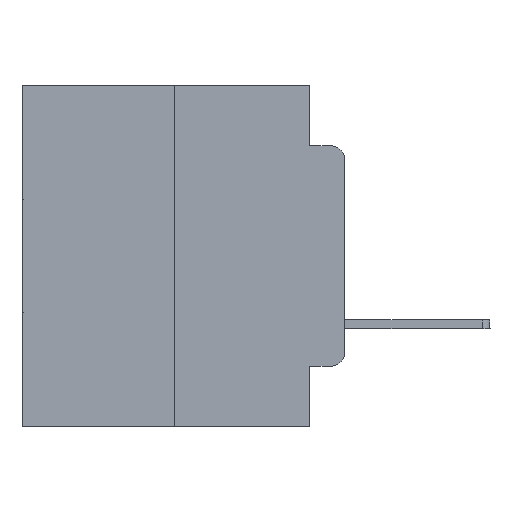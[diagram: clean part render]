
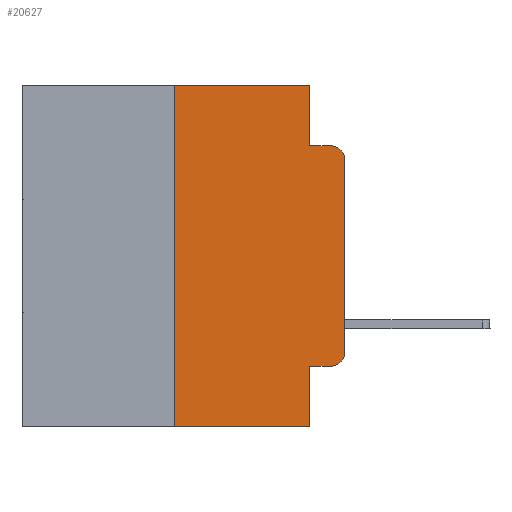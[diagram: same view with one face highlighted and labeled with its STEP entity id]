
A CAD part, left-side view. The second image highlights one B-rep face of the part: STEP entity #20627.
In plain terms, the highlighted planar face has unit normal (-1, 0, 0).
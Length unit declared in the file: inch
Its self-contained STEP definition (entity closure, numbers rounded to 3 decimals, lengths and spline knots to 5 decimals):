
#305 = ORIENTED_EDGE ( 'NONE', *, *, #5010, .T. ) ;
#1034 = ORIENTED_EDGE ( 'NONE', *, *, #11892, .F. ) ;
#1563 = CARTESIAN_POINT ( 'NONE',  ( 0., 0.02, -0.0885 ) ) ;
#1621 = ORIENTED_EDGE ( 'NONE', *, *, #8146, .T. ) ;
#1834 = ORIENTED_EDGE ( 'NONE', *, *, #20499, .T. ) ;
#1839 = VECTOR ( 'NONE', #17886, 39.37008 ) ;
#2283 = DIRECTION ( 'NONE',  ( 0., -1., 0. ) ) ;
#2463 = CARTESIAN_POINT ( 'NONE',  ( 0., 0.473, -0.5 ) ) ;
#2568 = CARTESIAN_POINT ( 'NONE',  ( 0., 0.25, 0. ) ) ;
#3021 = DIRECTION ( 'NONE',  ( 0., 0., 1. ) ) ;
#3445 = VERTEX_POINT ( 'NONE', #2568 ) ;
#3452 = DIRECTION ( 'NONE',  ( -1., 0., 0. ) ) ;
#4094 = LINE ( 'NONE', #2463, #12336 ) ;
#4284 = DIRECTION ( 'NONE',  ( 0., 0., -1. ) ) ;
#4393 = AXIS2_PLACEMENT_3D ( 'NONE', #25693, #23459, #19168 ) ;
#4467 = CARTESIAN_POINT ( 'NONE',  ( 0., 0.051, 0. ) ) ;
#4659 = CARTESIAN_POINT ( 'NONE',  ( 0., 0.25, -0.5 ) ) ;
#4790 = AXIS2_PLACEMENT_3D ( 'NONE', #21533, #3452, #23770 ) ;
#4793 = VERTEX_POINT ( 'NONE', #19976 ) ;
#5010 = EDGE_CURVE ( 'NONE', #17686, #23849, #25806, .T. ) ;
#5100 = VERTEX_POINT ( 'NONE', #1563 ) ;
#5243 = DIRECTION ( 'NONE',  ( 1., 0., 0. ) ) ;
#5441 = DIRECTION ( 'NONE',  ( 0., 0., -1. ) ) ;
#7052 = EDGE_CURVE ( 'NONE', #13944, #24182, #13206, .T. ) ;
#7358 = VECTOR ( 'NONE', #5441, 39.37008 ) ;
#7779 = CARTESIAN_POINT ( 'NONE',  ( 0., 0., -0.1085 ) ) ;
#7820 = VERTEX_POINT ( 'NONE', #4659 ) ;
#8146 = EDGE_CURVE ( 'NONE', #11826, #5100, #17295, .T. ) ;
#8486 = DIRECTION ( 'NONE',  ( 0., 0., 1. ) ) ;
#8573 = CARTESIAN_POINT ( 'NONE',  ( 0., 0.051, -0.4115 ) ) ;
#8834 = EDGE_CURVE ( 'NONE', #19646, #4793, #15980, .T. ) ;
#8929 = LINE ( 'NONE', #24575, #12171 ) ;
#9047 = CARTESIAN_POINT ( 'NONE',  ( 0., 0., 0. ) ) ;
#9195 = CARTESIAN_POINT ( 'NONE',  ( 0., 0.02, -0.4115 ) ) ;
#9342 = EDGE_CURVE ( 'NONE', #7820, #3445, #8929, .T. ) ;
#11826 = VERTEX_POINT ( 'NONE', #7779 ) ;
#11892 = EDGE_CURVE ( 'NONE', #3445, #13944, #18103, .T. ) ;
#12171 = VECTOR ( 'NONE', #8486, 39.37008 ) ;
#12336 = VECTOR ( 'NONE', #2283, 39.37008 ) ;
#12684 = ORIENTED_EDGE ( 'NONE', *, *, #9342, .F. ) ;
#12952 = LINE ( 'NONE', #15621, #24793 ) ;
#13206 = LINE ( 'NONE', #4467, #19613 ) ;
#13393 = DIRECTION ( 'NONE',  ( 0., 0., -1. ) ) ;
#13439 = CARTESIAN_POINT ( 'NONE',  ( 0., 0., -0.3915 ) ) ;
#13944 = VERTEX_POINT ( 'NONE', #15631 ) ;
#14394 = VECTOR ( 'NONE', #3021, 39.37008 ) ;
#14560 = FACE_OUTER_BOUND ( 'NONE', #25355, .T. ) ;
#15621 = CARTESIAN_POINT ( 'NONE',  ( 0., 0.051, -0.0885 ) ) ;
#15631 = CARTESIAN_POINT ( 'NONE',  ( 0., 0.051, 0. ) ) ;
#15738 = DIRECTION ( 'NONE',  ( 0., -1., 0. ) ) ;
#15980 = LINE ( 'NONE', #17700, #7358 ) ;
#16832 = VECTOR ( 'NONE', #15738, 39.37008 ) ;
#17137 = EDGE_CURVE ( 'NONE', #23849, #11826, #22411, .T. ) ;
#17243 = CARTESIAN_POINT ( 'NONE',  ( 0., 0.051, -0.0885 ) ) ;
#17295 = CIRCLE ( 'NONE', #4790, 0.02 ) ;
#17686 = VERTEX_POINT ( 'NONE', #9195 ) ;
#17700 = CARTESIAN_POINT ( 'NONE',  ( 0., 0.051, 0. ) ) ;
#17886 = DIRECTION ( 'NONE',  ( 0., -1., 0. ) ) ;
#17974 = ORIENTED_EDGE ( 'NONE', *, *, #7052, .F. ) ;
#18100 = LINE ( 'NONE', #21945, #1839 ) ;
#18103 = LINE ( 'NONE', #22184, #16832 ) ;
#19168 = DIRECTION ( 'NONE',  ( 0., 0., -1. ) ) ;
#19220 = PLANE ( 'NONE',  #23085 ) ;
#19613 = VECTOR ( 'NONE', #4284, 39.37008 ) ;
#19646 = VERTEX_POINT ( 'NONE', #8573 ) ;
#19653 = CARTESIAN_POINT ( 'NONE',  ( 0., 0.473, 0. ) ) ;
#19976 = CARTESIAN_POINT ( 'NONE',  ( 0., 0.051, -0.5 ) ) ;
#20499 = EDGE_CURVE ( 'NONE', #7820, #4793, #4094, .T. ) ;
#20627 = ADVANCED_FACE ( 'NONE', ( #14560 ), #19220, .F. ) ;
#20692 = EDGE_CURVE ( 'NONE', #24182, #5100, #12952, .T. ) ;
#21533 = CARTESIAN_POINT ( 'NONE',  ( 0., 0.02, -0.1085 ) ) ;
#21912 = ORIENTED_EDGE ( 'NONE', *, *, #8834, .F. ) ;
#21945 = CARTESIAN_POINT ( 'NONE',  ( 0., 0.051, -0.4115 ) ) ;
#22184 = CARTESIAN_POINT ( 'NONE',  ( 0., 0.473, 0. ) ) ;
#22411 = LINE ( 'NONE', #9047, #14394 ) ;
#23085 = AXIS2_PLACEMENT_3D ( 'NONE', #19653, #5243, #13393 ) ;
#23150 = ORIENTED_EDGE ( 'NONE', *, *, #17137, .T. ) ;
#23459 = DIRECTION ( 'NONE',  ( -1., 0., 0. ) ) ;
#23770 = DIRECTION ( 'NONE',  ( 0., 0., -1. ) ) ;
#23849 = VERTEX_POINT ( 'NONE', #13439 ) ;
#23898 = EDGE_CURVE ( 'NONE', #19646, #17686, #18100, .T. ) ;
#24182 = VERTEX_POINT ( 'NONE', #17243 ) ;
#24575 = CARTESIAN_POINT ( 'NONE',  ( 0., 0.25, 0. ) ) ;
#24793 = VECTOR ( 'NONE', #25663, 39.37008 ) ;
#25191 = ORIENTED_EDGE ( 'NONE', *, *, #20692, .F. ) ;
#25355 = EDGE_LOOP ( 'NONE', ( #23150, #1621, #25191, #17974, #1034, #12684, #1834, #21912, #25439, #305 ) ) ;
#25439 = ORIENTED_EDGE ( 'NONE', *, *, #23898, .T. ) ;
#25663 = DIRECTION ( 'NONE',  ( 0., -1., 0. ) ) ;
#25693 = CARTESIAN_POINT ( 'NONE',  ( 0., 0.02, -0.3915 ) ) ;
#25806 = CIRCLE ( 'NONE', #4393, 0.02 ) ;
